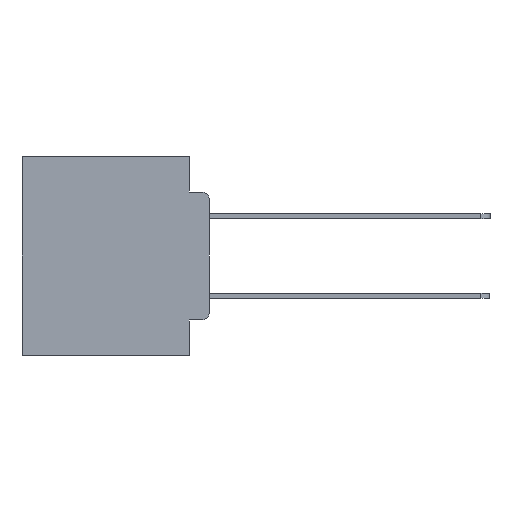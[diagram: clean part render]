
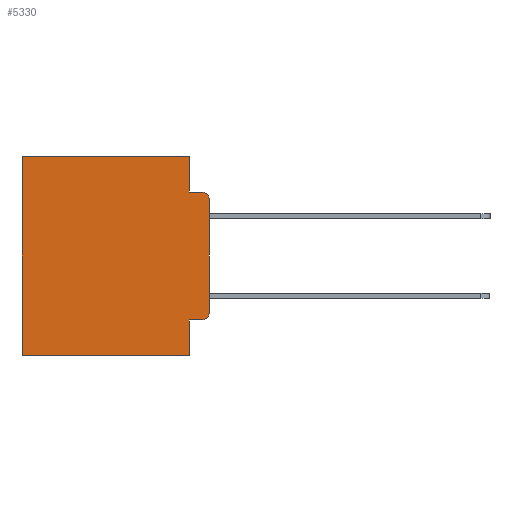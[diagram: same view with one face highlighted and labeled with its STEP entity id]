
A CAD part, left-side view. The second image highlights one B-rep face of the part: STEP entity #5330.
In plain terms, the highlighted planar face has unit normal (-1, 0, 0).
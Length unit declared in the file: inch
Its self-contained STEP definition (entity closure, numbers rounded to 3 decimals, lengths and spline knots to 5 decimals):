
#369 = CARTESIAN_POINT ( 'NONE',  ( 0.298, 0.051, 0. ) ) ;
#614 = DIRECTION ( 'NONE',  ( 0., 0., -1. ) ) ;
#1043 = CARTESIAN_POINT ( 'NONE',  ( 0.298, 0.051, -0.4115 ) ) ;
#1086 = CARTESIAN_POINT ( 'NONE',  ( 0.298, 0., -0.5 ) ) ;
#1255 = CARTESIAN_POINT ( 'NONE',  ( 0.298, 0.02, -0.1085 ) ) ;
#2040 = ORIENTED_EDGE ( 'NONE', *, *, #6916, .T. ) ;
#2253 = CARTESIAN_POINT ( 'NONE',  ( 0.298, 0.051, 0. ) ) ;
#2282 = DIRECTION ( 'NONE',  ( 0., 0., -1. ) ) ;
#3273 = CARTESIAN_POINT ( 'NONE',  ( 0.298, 0.051, 0. ) ) ;
#3367 = DIRECTION ( 'NONE',  ( 0., 0., -1. ) ) ;
#4295 = EDGE_CURVE ( 'NONE', #6839, #20711, #8498, .T. ) ;
#4348 = DIRECTION ( 'NONE',  ( 0., 0., -1. ) ) ;
#4566 = EDGE_CURVE ( 'NONE', #12934, #16897, #19109, .T. ) ;
#5314 = LINE ( 'NONE', #22225, #22215 ) ;
#5330 = ADVANCED_FACE ( 'NONE', ( #24139 ), #17585, .F. ) ;
#5424 = CARTESIAN_POINT ( 'NONE',  ( 0.298, 0.051, -0.5 ) ) ;
#5498 = DIRECTION ( 'NONE',  ( 0., -1., 0. ) ) ;
#5622 = ORIENTED_EDGE ( 'NONE', *, *, #5930, .T. ) ;
#5858 = VECTOR ( 'NONE', #23621, 39.37008 ) ;
#5930 = EDGE_CURVE ( 'NONE', #20711, #16530, #5314, .T. ) ;
#6255 = ORIENTED_EDGE ( 'NONE', *, *, #26295, .F. ) ;
#6618 = AXIS2_PLACEMENT_3D ( 'NONE', #11489, #19659, #7366 ) ;
#6705 = DIRECTION ( 'NONE',  ( 1., 0., 0. ) ) ;
#6818 = CARTESIAN_POINT ( 'NONE',  ( 0.298, 0., 0. ) ) ;
#6839 = VERTEX_POINT ( 'NONE', #369 ) ;
#6916 = EDGE_CURVE ( 'NONE', #10998, #10519, #17766, .T. ) ;
#7355 = VECTOR ( 'NONE', #5498, 39.37008 ) ;
#7366 = DIRECTION ( 'NONE',  ( 0., 0., -1. ) ) ;
#8289 = EDGE_CURVE ( 'NONE', #12934, #10998, #16123, .T. ) ;
#8498 = LINE ( 'NONE', #22051, #24132 ) ;
#8544 = VERTEX_POINT ( 'NONE', #8916 ) ;
#8787 = EDGE_LOOP ( 'NONE', ( #9094, #14572, #9754, #20636, #17306, #5622, #6255, #11675, #23140, #2040 ) ) ;
#8838 = DIRECTION ( 'NONE',  ( 0., 0., -1. ) ) ;
#8916 = CARTESIAN_POINT ( 'NONE',  ( 0.298, 0.051, -0.0885 ) ) ;
#9094 = ORIENTED_EDGE ( 'NONE', *, *, #19157, .F. ) ;
#9533 = CARTESIAN_POINT ( 'NONE',  ( 0.298, 0.02, -0.0885 ) ) ;
#9754 = ORIENTED_EDGE ( 'NONE', *, *, #14144, .F. ) ;
#9840 = CARTESIAN_POINT ( 'NONE',  ( 0.298, 0., -0.3915 ) ) ;
#9916 = CARTESIAN_POINT ( 'NONE',  ( 0.298, 0., 0. ) ) ;
#10033 = EDGE_CURVE ( 'NONE', #6839, #8544, #24567, .T. ) ;
#10519 = VERTEX_POINT ( 'NONE', #9840 ) ;
#10998 = VERTEX_POINT ( 'NONE', #21157 ) ;
#11489 = CARTESIAN_POINT ( 'NONE',  ( 0.298, 0.02, -0.3915 ) ) ;
#11675 = ORIENTED_EDGE ( 'NONE', *, *, #4566, .F. ) ;
#12934 = VERTEX_POINT ( 'NONE', #1043 ) ;
#13738 = VECTOR ( 'NONE', #2282, 39.37008 ) ;
#14144 = EDGE_CURVE ( 'NONE', #8544, #21165, #23615, .T. ) ;
#14318 = CARTESIAN_POINT ( 'NONE',  ( 0.298, 0.473, 0. ) ) ;
#14555 = CIRCLE ( 'NONE', #23424, 0.02 ) ;
#14572 = ORIENTED_EDGE ( 'NONE', *, *, #23659, .T. ) ;
#14695 = VERTEX_POINT ( 'NONE', #19509 ) ;
#15679 = DIRECTION ( 'NONE',  ( -1., 0., 0. ) ) ;
#15709 = CARTESIAN_POINT ( 'NONE',  ( 0.298, 0.051, -0.0885 ) ) ;
#16122 = LINE ( 'NONE', #6818, #26290 ) ;
#16123 = LINE ( 'NONE', #26000, #5858 ) ;
#16530 = VERTEX_POINT ( 'NONE', #20632 ) ;
#16897 = VERTEX_POINT ( 'NONE', #5424 ) ;
#17306 = ORIENTED_EDGE ( 'NONE', *, *, #4295, .T. ) ;
#17585 = PLANE ( 'NONE',  #21939 ) ;
#17606 = DIRECTION ( 'NONE',  ( 0., 1., 0. ) ) ;
#17766 = CIRCLE ( 'NONE', #6618, 0.02 ) ;
#18278 = DIRECTION ( 'NONE',  ( 0., 1., 0. ) ) ;
#18287 = LINE ( 'NONE', #1086, #22970 ) ;
#19109 = LINE ( 'NONE', #3273, #23792 ) ;
#19157 = EDGE_CURVE ( 'NONE', #14695, #10519, #16122, .T. ) ;
#19509 = CARTESIAN_POINT ( 'NONE',  ( 0.298, 0., -0.1085 ) ) ;
#19659 = DIRECTION ( 'NONE',  ( -1., 0., 0. ) ) ;
#20632 = CARTESIAN_POINT ( 'NONE',  ( 0.298, 0.473, -0.5 ) ) ;
#20636 = ORIENTED_EDGE ( 'NONE', *, *, #10033, .F. ) ;
#20711 = VERTEX_POINT ( 'NONE', #14318 ) ;
#21157 = CARTESIAN_POINT ( 'NONE',  ( 0.298, 0.02, -0.4115 ) ) ;
#21165 = VERTEX_POINT ( 'NONE', #9533 ) ;
#21939 = AXIS2_PLACEMENT_3D ( 'NONE', #9916, #6705, #24103 ) ;
#22051 = CARTESIAN_POINT ( 'NONE',  ( 0.298, 0., 0. ) ) ;
#22215 = VECTOR ( 'NONE', #4348, 39.37008 ) ;
#22225 = CARTESIAN_POINT ( 'NONE',  ( 0.298, 0.473, 0. ) ) ;
#22970 = VECTOR ( 'NONE', #17606, 39.37008 ) ;
#23140 = ORIENTED_EDGE ( 'NONE', *, *, #8289, .T. ) ;
#23424 = AXIS2_PLACEMENT_3D ( 'NONE', #1255, #15679, #3367 ) ;
#23615 = LINE ( 'NONE', #15709, #7355 ) ;
#23621 = DIRECTION ( 'NONE',  ( 0., -1., 0. ) ) ;
#23659 = EDGE_CURVE ( 'NONE', #14695, #21165, #14555, .T. ) ;
#23792 = VECTOR ( 'NONE', #8838, 39.37008 ) ;
#24103 = DIRECTION ( 'NONE',  ( 0., 0., -1. ) ) ;
#24132 = VECTOR ( 'NONE', #18278, 39.37008 ) ;
#24139 = FACE_OUTER_BOUND ( 'NONE', #8787, .T. ) ;
#24567 = LINE ( 'NONE', #2253, #13738 ) ;
#26000 = CARTESIAN_POINT ( 'NONE',  ( 0.298, 0.051, -0.4115 ) ) ;
#26290 = VECTOR ( 'NONE', #614, 39.37008 ) ;
#26295 = EDGE_CURVE ( 'NONE', #16897, #16530, #18287, .T. ) ;
